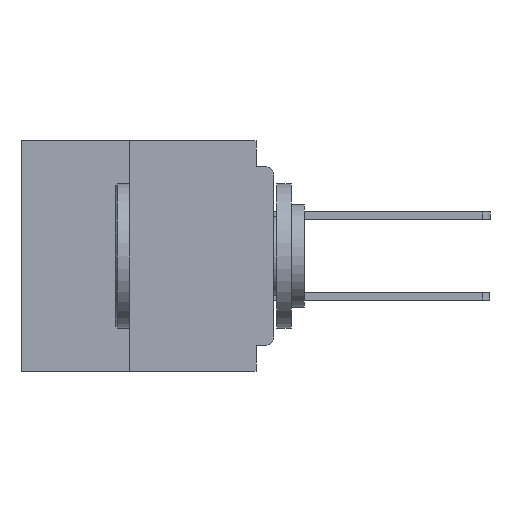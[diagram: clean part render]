
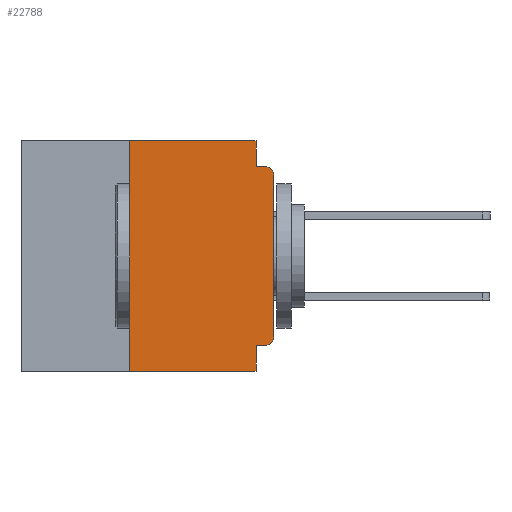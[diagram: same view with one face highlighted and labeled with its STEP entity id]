
A CAD part, left-side view. The second image highlights one B-rep face of the part: STEP entity #22788.
In plain terms, the highlighted planar face has unit normal (-1, 0, 0).
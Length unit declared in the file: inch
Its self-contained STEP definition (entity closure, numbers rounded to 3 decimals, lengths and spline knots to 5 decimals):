
#1 = CARTESIAN_POINT ( 'NONE',  ( 0., 0.437, 0. ) ) ;
#2112 = VECTOR ( 'NONE', #26335, 39.37008 ) ;
#2122 = VERTEX_POINT ( 'NONE', #14084 ) ;
#4298 = VECTOR ( 'NONE', #48538, 39.37008 ) ;
#4488 = DIRECTION ( 'NONE',  ( 0., 0., -1. ) ) ;
#4632 = FACE_OUTER_BOUND ( 'NONE', #36217, .T. ) ;
#4681 = CIRCLE ( 'NONE', #15582, 0.015 ) ;
#7660 = EDGE_CURVE ( 'NONE', #8947, #10472, #33917, .T. ) ;
#8947 = VERTEX_POINT ( 'NONE', #31003 ) ;
#9602 = DIRECTION ( 'NONE',  ( 0., 1., 0. ) ) ;
#10338 = DIRECTION ( 'NONE',  ( 0., -1., 0. ) ) ;
#10472 = VERTEX_POINT ( 'NONE', #19430 ) ;
#10640 = VERTEX_POINT ( 'NONE', #34191 ) ;
#12343 = DIRECTION ( 'NONE',  ( -1., 0., 0. ) ) ;
#12663 = CARTESIAN_POINT ( 'NONE',  ( 0., 0., -0.06 ) ) ;
#13236 = ORIENTED_EDGE ( 'NONE', *, *, #19456, .T. ) ;
#14084 = CARTESIAN_POINT ( 'NONE',  ( 0., 0.031, 0. ) ) ;
#15552 = LINE ( 'NONE', #18659, #26133 ) ;
#15582 = AXIS2_PLACEMENT_3D ( 'NONE', #16323, #47890, #20822 ) ;
#16304 = LINE ( 'NONE', #21455, #4298 ) ;
#16323 = CARTESIAN_POINT ( 'NONE',  ( 0., 0.015, -0.06 ) ) ;
#17556 = ORIENTED_EDGE ( 'NONE', *, *, #47509, .F. ) ;
#18659 = CARTESIAN_POINT ( 'NONE',  ( 0., 0., -0.355 ) ) ;
#18909 = EDGE_CURVE ( 'NONE', #45578, #48146, #28930, .T. ) ;
#19430 = CARTESIAN_POINT ( 'NONE',  ( 0., 0.015, -0.045 ) ) ;
#19456 = EDGE_CURVE ( 'NONE', #27437, #45578, #33810, .T. ) ;
#19584 = CARTESIAN_POINT ( 'NONE',  ( 0., 0.25, -0.4 ) ) ;
#19653 = LINE ( 'NONE', #19584, #31626 ) ;
#20328 = CARTESIAN_POINT ( 'NONE',  ( 0., 0.031, -0.355 ) ) ;
#20506 = VECTOR ( 'NONE', #10338, 39.37008 ) ;
#20822 = DIRECTION ( 'NONE',  ( 0., 0., -1. ) ) ;
#20990 = EDGE_CURVE ( 'NONE', #10640, #53540, #19653, .T. ) ;
#21455 = CARTESIAN_POINT ( 'NONE',  ( 0., 0.437, 0. ) ) ;
#21640 = CARTESIAN_POINT ( 'NONE',  ( 0., 0., 0. ) ) ;
#21790 = CARTESIAN_POINT ( 'NONE',  ( 0., 0.031, 0. ) ) ;
#22336 = EDGE_CURVE ( 'NONE', #48146, #10472, #4681, .T. ) ;
#22788 = ADVANCED_FACE ( 'NONE', ( #4632 ), #26954, .F. ) ;
#24286 = ORIENTED_EDGE ( 'NONE', *, *, #18909, .T. ) ;
#24406 = EDGE_CURVE ( 'NONE', #39787, #36974, #48304, .T. ) ;
#24626 = DIRECTION ( 'NONE',  ( 0., 0., -1. ) ) ;
#24920 = CARTESIAN_POINT ( 'NONE',  ( 0., 0.031, -0.4 ) ) ;
#26133 = VECTOR ( 'NONE', #9602, 39.37008 ) ;
#26335 = DIRECTION ( 'NONE',  ( 0., 0., -1. ) ) ;
#26954 = PLANE ( 'NONE',  #53783 ) ;
#27134 = DIRECTION ( 'NONE',  ( 0., -1., 0. ) ) ;
#27437 = VERTEX_POINT ( 'NONE', #41720 ) ;
#27529 = VECTOR ( 'NONE', #39837, 39.37008 ) ;
#28243 = CARTESIAN_POINT ( 'NONE',  ( 0., 0., -0.045 ) ) ;
#28930 = LINE ( 'NONE', #21640, #27529 ) ;
#29837 = ORIENTED_EDGE ( 'NONE', *, *, #37093, .F. ) ;
#30732 = CARTESIAN_POINT ( 'NONE',  ( 0., 0.25, 0. ) ) ;
#31003 = CARTESIAN_POINT ( 'NONE',  ( 0., 0.031, -0.045 ) ) ;
#31455 = DIRECTION ( 'NONE',  ( 1., 0., 0. ) ) ;
#31626 = VECTOR ( 'NONE', #46628, 39.37008 ) ;
#33531 = ORIENTED_EDGE ( 'NONE', *, *, #20990, .F. ) ;
#33810 = CIRCLE ( 'NONE', #44220, 0.015 ) ;
#33917 = LINE ( 'NONE', #28243, #20506 ) ;
#34191 = CARTESIAN_POINT ( 'NONE',  ( 0., 0.25, -0.4 ) ) ;
#36217 = EDGE_LOOP ( 'NONE', ( #24286, #40319, #53302, #17556, #46944, #33531, #49503, #40792, #29837, #13236 ) ) ;
#36260 = VECTOR ( 'NONE', #24626, 39.37008 ) ;
#36974 = VERTEX_POINT ( 'NONE', #24920 ) ;
#37093 = EDGE_CURVE ( 'NONE', #27437, #39787, #15552, .T. ) ;
#38093 = LINE ( 'NONE', #21790, #2112 ) ;
#39267 = CARTESIAN_POINT ( 'NONE',  ( 0., 0., -0.34 ) ) ;
#39371 = CARTESIAN_POINT ( 'NONE',  ( 0., 0.015, -0.34 ) ) ;
#39787 = VERTEX_POINT ( 'NONE', #20328 ) ;
#39837 = DIRECTION ( 'NONE',  ( 0., 0., 1. ) ) ;
#39952 = LINE ( 'NONE', #49683, #53332 ) ;
#40319 = ORIENTED_EDGE ( 'NONE', *, *, #22336, .T. ) ;
#40792 = ORIENTED_EDGE ( 'NONE', *, *, #24406, .F. ) ;
#41720 = CARTESIAN_POINT ( 'NONE',  ( 0., 0.015, -0.355 ) ) ;
#42624 = CARTESIAN_POINT ( 'NONE',  ( 0., 0.031, -0.4 ) ) ;
#43925 = DIRECTION ( 'NONE',  ( 0., 0., -1. ) ) ;
#44220 = AXIS2_PLACEMENT_3D ( 'NONE', #39371, #12343, #43925 ) ;
#45578 = VERTEX_POINT ( 'NONE', #39267 ) ;
#46628 = DIRECTION ( 'NONE',  ( 0., 0., 1. ) ) ;
#46802 = EDGE_CURVE ( 'NONE', #53540, #2122, #16304, .T. ) ;
#46944 = ORIENTED_EDGE ( 'NONE', *, *, #46802, .F. ) ;
#47509 = EDGE_CURVE ( 'NONE', #2122, #8947, #38093, .T. ) ;
#47890 = DIRECTION ( 'NONE',  ( -1., 0., 0. ) ) ;
#48146 = VERTEX_POINT ( 'NONE', #12663 ) ;
#48304 = LINE ( 'NONE', #42624, #36260 ) ;
#48538 = DIRECTION ( 'NONE',  ( 0., -1., 0. ) ) ;
#49503 = ORIENTED_EDGE ( 'NONE', *, *, #57451, .T. ) ;
#49683 = CARTESIAN_POINT ( 'NONE',  ( 0., 0.437, -0.4 ) ) ;
#53302 = ORIENTED_EDGE ( 'NONE', *, *, #7660, .F. ) ;
#53332 = VECTOR ( 'NONE', #27134, 39.37008 ) ;
#53540 = VERTEX_POINT ( 'NONE', #30732 ) ;
#53783 = AXIS2_PLACEMENT_3D ( 'NONE', #1, #31455, #4488 ) ;
#57451 = EDGE_CURVE ( 'NONE', #10640, #36974, #39952, .T. ) ;
